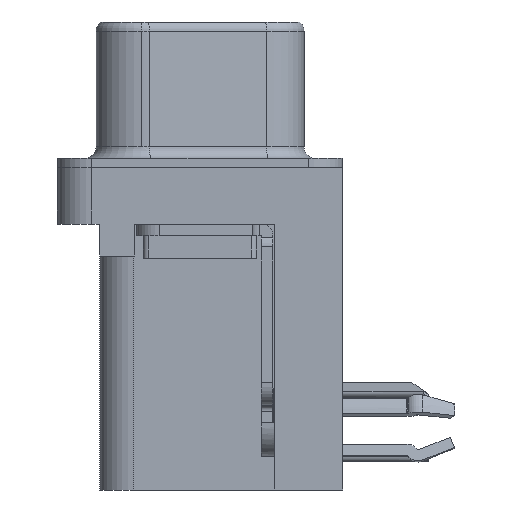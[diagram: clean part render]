
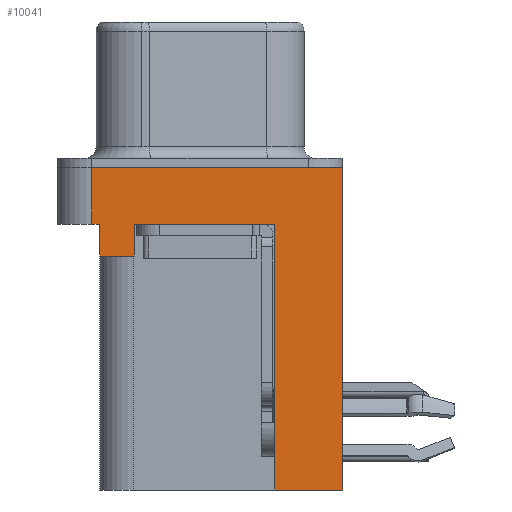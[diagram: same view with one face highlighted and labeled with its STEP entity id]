
A CAD part, left-side view. The second image highlights one B-rep face of the part: STEP entity #10041.
In plain terms, the highlighted planar face has unit normal (-1, 0, 0).
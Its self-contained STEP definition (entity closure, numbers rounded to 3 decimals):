
#111 = CARTESIAN_POINT ( 'NONE',  ( -2.935, -6.275, -14.2 ) ) ;
#753 = DIRECTION ( 'NONE',  ( 0., -1., 0. ) ) ;
#809 = EDGE_CURVE ( 'NONE', #5160, #2017, #12312, .T. ) ;
#964 = DIRECTION ( 'NONE',  ( 0., -1., 0. ) ) ;
#1114 = ORIENTED_EDGE ( 'NONE', *, *, #16409, .F. ) ;
#1220 = CARTESIAN_POINT ( 'NONE',  ( -2.935, 4.425, -3.9 ) ) ;
#1401 = DIRECTION ( 'NONE',  ( 0., 1., 0. ) ) ;
#1477 = CARTESIAN_POINT ( 'NONE',  ( -2.935, 4.775, 0. ) ) ;
#2017 = VERTEX_POINT ( 'NONE', #15769 ) ;
#2417 = VERTEX_POINT ( 'NONE', #111 ) ;
#2620 = CARTESIAN_POINT ( 'NONE',  ( -2.935, 2.895, -3.9 ) ) ;
#2753 = EDGE_CURVE ( 'NONE', #15804, #16063, #14139, .T. ) ;
#3274 = EDGE_CURVE ( 'NONE', #2417, #17127, #16959, .T. ) ;
#3664 = EDGE_CURVE ( 'NONE', #2417, #9011, #5774, .T. ) ;
#3719 = CARTESIAN_POINT ( 'NONE',  ( -2.935, -6.275, 0. ) ) ;
#3819 = CARTESIAN_POINT ( 'NONE',  ( -2.935, 4.775, -2.5 ) ) ;
#4144 = CARTESIAN_POINT ( 'NONE',  ( -2.935, -3.295, -14.2 ) ) ;
#4188 = DIRECTION ( 'NONE',  ( 0., 0., 1. ) ) ;
#4228 = ORIENTED_EDGE ( 'NONE', *, *, #14221, .T. ) ;
#4873 = DIRECTION ( 'NONE',  ( 0., 0., 1. ) ) ;
#4887 = VERTEX_POINT ( 'NONE', #15422 ) ;
#4988 = CARTESIAN_POINT ( 'NONE',  ( -2.935, -6.275, -2.5 ) ) ;
#4997 = DIRECTION ( 'NONE',  ( -1., 0., 0. ) ) ;
#5101 = VECTOR ( 'NONE', #4873, 1000. ) ;
#5104 = ORIENTED_EDGE ( 'NONE', *, *, #6486, .F. ) ;
#5160 = VERTEX_POINT ( 'NONE', #10427 ) ;
#5509 = DIRECTION ( 'NONE',  ( 0., 0., 1. ) ) ;
#5580 = LINE ( 'NONE', #18117, #6303 ) ;
#5774 = LINE ( 'NONE', #11340, #13840 ) ;
#6124 = DIRECTION ( 'NONE',  ( 0., 0., 1. ) ) ;
#6300 = ORIENTED_EDGE ( 'NONE', *, *, #3274, .F. ) ;
#6303 = VECTOR ( 'NONE', #16815, 1000. ) ;
#6486 = EDGE_CURVE ( 'NONE', #16633, #9011, #16435, .T. ) ;
#7499 = EDGE_CURVE ( 'NONE', #5160, #16633, #10899, .T. ) ;
#7585 = LINE ( 'NONE', #13219, #5101 ) ;
#7666 = ORIENTED_EDGE ( 'NONE', *, *, #7499, .F. ) ;
#7800 = PLANE ( 'NONE',  #12007 ) ;
#8008 = EDGE_CURVE ( 'NONE', #17127, #4887, #5580, .T. ) ;
#8420 = CARTESIAN_POINT ( 'NONE',  ( -2.935, -6.275, 0. ) ) ;
#9011 = VERTEX_POINT ( 'NONE', #8420 ) ;
#9068 = LINE ( 'NONE', #9154, #15552 ) ;
#9154 = CARTESIAN_POINT ( 'NONE',  ( -2.935, -6.275, -2.5 ) ) ;
#9777 = CARTESIAN_POINT ( 'NONE',  ( -2.935, 2.895, -2.5 ) ) ;
#10041 = ADVANCED_FACE ( 'NONE', ( #17803 ), #7800, .T. ) ;
#10370 = ORIENTED_EDGE ( 'NONE', *, *, #11944, .T. ) ;
#10427 = CARTESIAN_POINT ( 'NONE',  ( -2.935, 4.775, -2.5 ) ) ;
#10710 = VECTOR ( 'NONE', #13202, 1000. ) ;
#10899 = LINE ( 'NONE', #3819, #17553 ) ;
#11279 = LINE ( 'NONE', #2620, #15338 ) ;
#11340 = CARTESIAN_POINT ( 'NONE',  ( -2.935, -6.275, -2.5 ) ) ;
#11854 = CARTESIAN_POINT ( 'NONE',  ( -2.935, 2.895, -3.9 ) ) ;
#11944 = EDGE_CURVE ( 'NONE', #13447, #4887, #9068, .T. ) ;
#12007 = AXIS2_PLACEMENT_3D ( 'NONE', #14557, #4997, #6124 ) ;
#12312 = LINE ( 'NONE', #4988, #15707 ) ;
#13194 = ORIENTED_EDGE ( 'NONE', *, *, #809, .T. ) ;
#13202 = DIRECTION ( 'NONE',  ( 0., -1., 0. ) ) ;
#13219 = CARTESIAN_POINT ( 'NONE',  ( -2.935, 4.425, -3.9 ) ) ;
#13447 = VERTEX_POINT ( 'NONE', #9777 ) ;
#13840 = VECTOR ( 'NONE', #4188, 1000. ) ;
#14139 = LINE ( 'NONE', #1220, #17706 ) ;
#14188 = CARTESIAN_POINT ( 'NONE',  ( -2.935, -3.295, -14.2 ) ) ;
#14221 = EDGE_CURVE ( 'NONE', #15804, #13447, #11279, .T. ) ;
#14248 = VECTOR ( 'NONE', #18275, 1000. ) ;
#14557 = CARTESIAN_POINT ( 'NONE',  ( -2.935, -6.275, -2.5 ) ) ;
#15100 = EDGE_LOOP ( 'NONE', ( #5104, #7666, #13194, #1114, #17107, #4228, #10370, #18099, #6300, #15898 ) ) ;
#15338 = VECTOR ( 'NONE', #17139, 1000. ) ;
#15422 = CARTESIAN_POINT ( 'NONE',  ( -2.935, -3.295, -2.5 ) ) ;
#15552 = VECTOR ( 'NONE', #753, 1000. ) ;
#15707 = VECTOR ( 'NONE', #964, 1000. ) ;
#15769 = CARTESIAN_POINT ( 'NONE',  ( -2.935, 4.425, -2.5 ) ) ;
#15804 = VERTEX_POINT ( 'NONE', #11854 ) ;
#15898 = ORIENTED_EDGE ( 'NONE', *, *, #3664, .T. ) ;
#16063 = VERTEX_POINT ( 'NONE', #17980 ) ;
#16409 = EDGE_CURVE ( 'NONE', #16063, #2017, #7585, .T. ) ;
#16435 = LINE ( 'NONE', #3719, #10710 ) ;
#16633 = VERTEX_POINT ( 'NONE', #1477 ) ;
#16815 = DIRECTION ( 'NONE',  ( 0., 0., 1. ) ) ;
#16959 = LINE ( 'NONE', #4144, #14248 ) ;
#17107 = ORIENTED_EDGE ( 'NONE', *, *, #2753, .F. ) ;
#17127 = VERTEX_POINT ( 'NONE', #14188 ) ;
#17139 = DIRECTION ( 'NONE',  ( 0., 0., 1. ) ) ;
#17553 = VECTOR ( 'NONE', #5509, 1000. ) ;
#17706 = VECTOR ( 'NONE', #1401, 1000. ) ;
#17803 = FACE_OUTER_BOUND ( 'NONE', #15100, .T. ) ;
#17980 = CARTESIAN_POINT ( 'NONE',  ( -2.935, 4.425, -3.9 ) ) ;
#18099 = ORIENTED_EDGE ( 'NONE', *, *, #8008, .F. ) ;
#18117 = CARTESIAN_POINT ( 'NONE',  ( -2.935, -3.295, -14.2 ) ) ;
#18275 = DIRECTION ( 'NONE',  ( 0., 1., 0. ) ) ;
